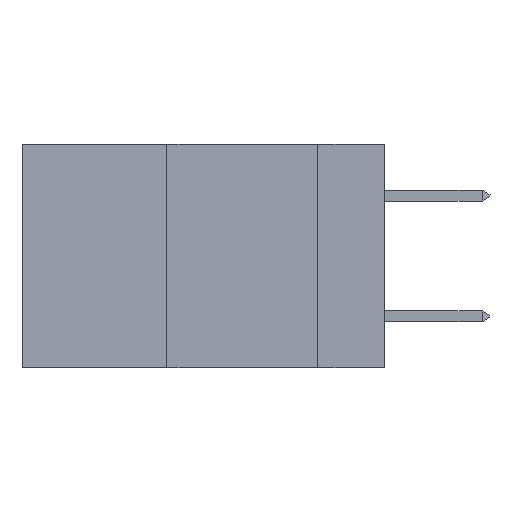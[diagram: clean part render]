
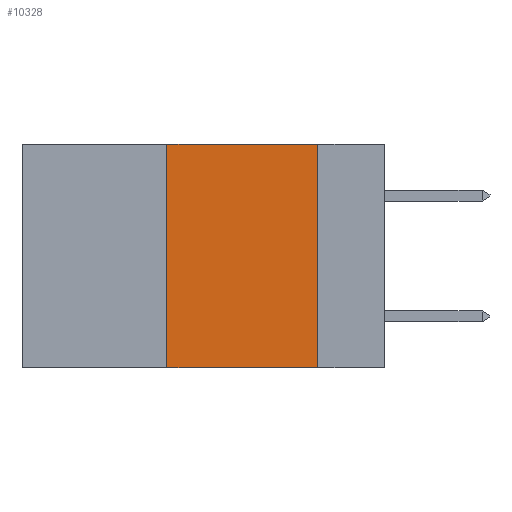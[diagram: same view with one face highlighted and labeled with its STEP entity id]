
A CAD part, left-side view. The second image highlights one B-rep face of the part: STEP entity #10328.
In plain terms, the highlighted planar face has unit normal (-1, 0, 0).
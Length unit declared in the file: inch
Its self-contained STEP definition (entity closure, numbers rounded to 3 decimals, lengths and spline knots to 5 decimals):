
#642 = VECTOR ( 'NONE', #8668, 39.37008 ) ;
#836 = VECTOR ( 'NONE', #2426, 39.37008 ) ;
#1228 = CARTESIAN_POINT ( 'NONE',  ( 0., 0.36, -0.37 ) ) ;
#1497 = LINE ( 'NONE', #11447, #836 ) ;
#1702 = VERTEX_POINT ( 'NONE', #5847 ) ;
#1729 = CARTESIAN_POINT ( 'NONE',  ( 0., 0.36, 0. ) ) ;
#2007 = VERTEX_POINT ( 'NONE', #1228 ) ;
#2109 = EDGE_CURVE ( 'NONE', #8667, #1702, #10805, .T. ) ;
#2426 = DIRECTION ( 'NONE',  ( 0., 0., 1. ) ) ;
#2599 = DIRECTION ( 'NONE',  ( 0., 0., -1. ) ) ;
#2699 = EDGE_CURVE ( 'NONE', #1702, #9830, #12110, .T. ) ;
#2716 = EDGE_CURVE ( 'NONE', #2007, #8667, #1497, .T. ) ;
#2717 = EDGE_CURVE ( 'NONE', #2007, #9830, #3586, .T. ) ;
#3586 = LINE ( 'NONE', #8522, #8658 ) ;
#4010 = ORIENTED_EDGE ( 'NONE', *, *, #2699, .F. ) ;
#4220 = AXIS2_PLACEMENT_3D ( 'NONE', #7621, #8655, #2599 ) ;
#5617 = PLANE ( 'NONE',  #4220 ) ;
#5847 = CARTESIAN_POINT ( 'NONE',  ( 0., 0.11, 0. ) ) ;
#6612 = VECTOR ( 'NONE', #12302, 39.37008 ) ;
#7293 = ORIENTED_EDGE ( 'NONE', *, *, #2109, .F. ) ;
#7338 = ORIENTED_EDGE ( 'NONE', *, *, #2717, .T. ) ;
#7621 = CARTESIAN_POINT ( 'NONE',  ( 0., 0.6, 0. ) ) ;
#8092 = EDGE_LOOP ( 'NONE', ( #4010, #7293, #9114, #7338 ) ) ;
#8522 = CARTESIAN_POINT ( 'NONE',  ( 0., 0.6, -0.37 ) ) ;
#8655 = DIRECTION ( 'NONE',  ( 1., 0., 0. ) ) ;
#8658 = VECTOR ( 'NONE', #9558, 39.37008 ) ;
#8667 = VERTEX_POINT ( 'NONE', #1729 ) ;
#8668 = DIRECTION ( 'NONE',  ( 0., -1., 0. ) ) ;
#9114 = ORIENTED_EDGE ( 'NONE', *, *, #2716, .F. ) ;
#9354 = FACE_OUTER_BOUND ( 'NONE', #8092, .T. ) ;
#9465 = CARTESIAN_POINT ( 'NONE',  ( 0., 0.11, 0. ) ) ;
#9558 = DIRECTION ( 'NONE',  ( 0., -1., 0. ) ) ;
#9830 = VERTEX_POINT ( 'NONE', #10712 ) ;
#10328 = ADVANCED_FACE ( 'NONE', ( #9354 ), #5617, .F. ) ;
#10712 = CARTESIAN_POINT ( 'NONE',  ( 0., 0.11, -0.37 ) ) ;
#10805 = LINE ( 'NONE', #11697, #642 ) ;
#11447 = CARTESIAN_POINT ( 'NONE',  ( 0., 0.36, 0. ) ) ;
#11697 = CARTESIAN_POINT ( 'NONE',  ( 0., 0.6, 0. ) ) ;
#12110 = LINE ( 'NONE', #9465, #6612 ) ;
#12302 = DIRECTION ( 'NONE',  ( 0., 0., -1. ) ) ;
